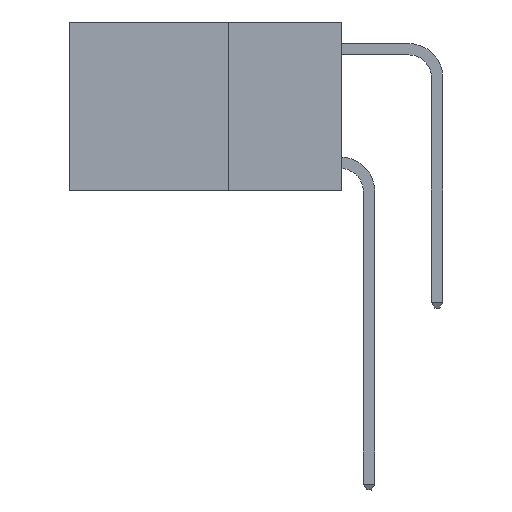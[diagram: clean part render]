
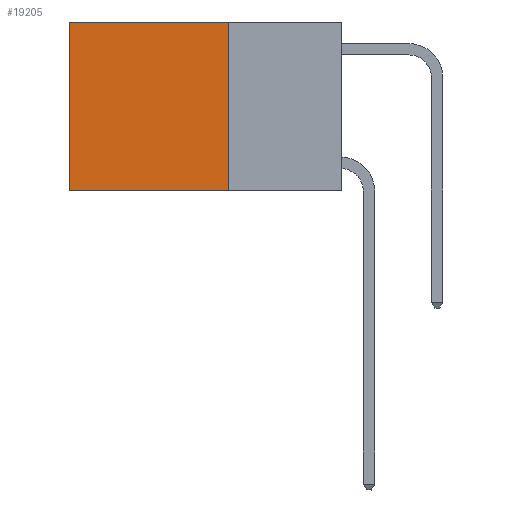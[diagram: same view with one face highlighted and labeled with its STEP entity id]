
A CAD part, left-side view. The second image highlights one B-rep face of the part: STEP entity #19205.
In plain terms, the highlighted planar face has unit normal (-1, 0, 0).
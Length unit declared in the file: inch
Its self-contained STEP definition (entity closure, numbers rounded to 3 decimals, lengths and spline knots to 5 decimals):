
#605 = DIRECTION ( 'NONE',  ( 0., 0., -1. ) ) ;
#814 = ORIENTED_EDGE ( 'NONE', *, *, #18345, .F. ) ;
#1023 = PLANE ( 'NONE',  #18295 ) ;
#1037 = VECTOR ( 'NONE', #14753, 39.37008 ) ;
#1105 = VERTEX_POINT ( 'NONE', #11277 ) ;
#1107 = ORIENTED_EDGE ( 'NONE', *, *, #17158, .T. ) ;
#1613 = ORIENTED_EDGE ( 'NONE', *, *, #19044, .F. ) ;
#2631 = VECTOR ( 'NONE', #16778, 39.37008 ) ;
#2648 = DIRECTION ( 'NONE',  ( 1., 0., 0. ) ) ;
#3390 = LINE ( 'NONE', #20120, #7211 ) ;
#4486 = VECTOR ( 'NONE', #7206, 39.37008 ) ;
#4649 = ORIENTED_EDGE ( 'NONE', *, *, #20086, .T. ) ;
#4652 = FACE_OUTER_BOUND ( 'NONE', #20919, .T. ) ;
#5323 = VERTEX_POINT ( 'NONE', #11279 ) ;
#7206 = DIRECTION ( 'NONE',  ( 0., 0., -1. ) ) ;
#7211 = VECTOR ( 'NONE', #605, 39.37008 ) ;
#11277 = CARTESIAN_POINT ( 'NONE',  ( 0.2625, 0.6, -0.37 ) ) ;
#11279 = CARTESIAN_POINT ( 'NONE',  ( 0.2625, 0.25, 0. ) ) ;
#11679 = VERTEX_POINT ( 'NONE', #19487 ) ;
#12454 = CARTESIAN_POINT ( 'NONE',  ( 0.2625, 0.25, 0. ) ) ;
#13073 = CARTESIAN_POINT ( 'NONE',  ( 0.2625, 0.25, 0. ) ) ;
#13200 = LINE ( 'NONE', #20162, #4486 ) ;
#14111 = LINE ( 'NONE', #13073, #1037 ) ;
#14131 = DIRECTION ( 'NONE',  ( 0., 0., -1. ) ) ;
#14753 = DIRECTION ( 'NONE',  ( 0., 1., 0. ) ) ;
#15147 = CARTESIAN_POINT ( 'NONE',  ( 0.2625, 0.25, -0.37 ) ) ;
#16282 = CARTESIAN_POINT ( 'NONE',  ( 0.2625, 0.6, 0. ) ) ;
#16778 = DIRECTION ( 'NONE',  ( 0., 1., 0. ) ) ;
#17158 = EDGE_CURVE ( 'NONE', #19453, #1105, #13200, .T. ) ;
#18295 = AXIS2_PLACEMENT_3D ( 'NONE', #12454, #2648, #14131 ) ;
#18345 = EDGE_CURVE ( 'NONE', #11679, #1105, #19996, .T. ) ;
#19044 = EDGE_CURVE ( 'NONE', #5323, #11679, #3390, .T. ) ;
#19205 = ADVANCED_FACE ( 'NONE', ( #4652 ), #1023, .F. ) ;
#19453 = VERTEX_POINT ( 'NONE', #16282 ) ;
#19487 = CARTESIAN_POINT ( 'NONE',  ( 0.2625, 0.25, -0.37 ) ) ;
#19996 = LINE ( 'NONE', #15147, #2631 ) ;
#20086 = EDGE_CURVE ( 'NONE', #5323, #19453, #14111, .T. ) ;
#20120 = CARTESIAN_POINT ( 'NONE',  ( 0.2625, 0.25, 0. ) ) ;
#20162 = CARTESIAN_POINT ( 'NONE',  ( 0.2625, 0.6, 0. ) ) ;
#20919 = EDGE_LOOP ( 'NONE', ( #1107, #814, #1613, #4649 ) ) ;
